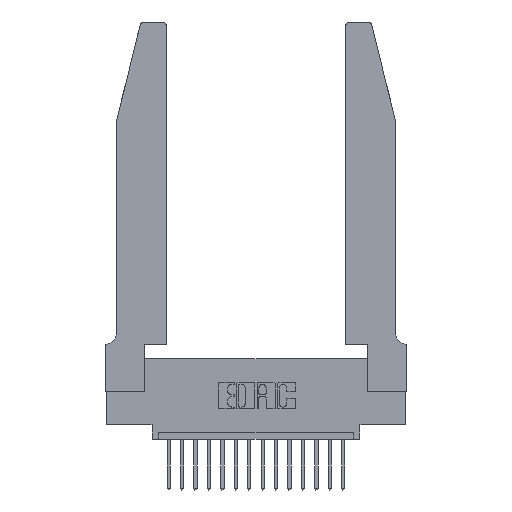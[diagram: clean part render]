
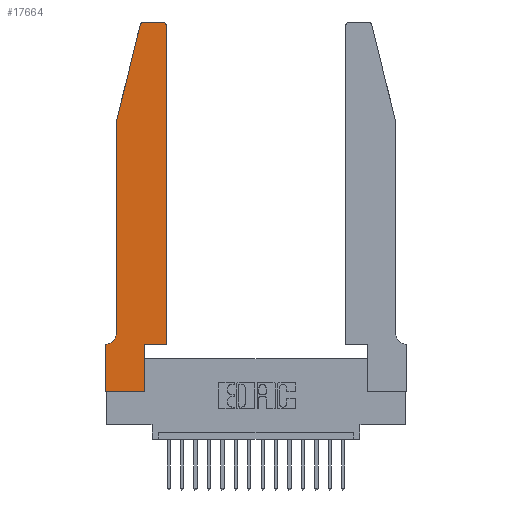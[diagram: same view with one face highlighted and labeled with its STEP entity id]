
A CAD part, top view. The second image highlights one B-rep face of the part: STEP entity #17664.
In plain terms, the highlighted planar face has unit normal (0, 0, 1).
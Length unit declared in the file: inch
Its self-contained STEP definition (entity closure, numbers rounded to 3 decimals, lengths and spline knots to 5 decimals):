
#41 = CARTESIAN_POINT ( 'NONE',  ( 0.0055, 0.35, 0.37 ) ) ;
#336 = DIRECTION ( 'NONE',  ( -1., 0., 0. ) ) ;
#634 = EDGE_CURVE ( 'NONE', #5556, #18562, #10754, .T. ) ;
#783 = EDGE_CURVE ( 'NONE', #3052, #7503, #3589, .T. ) ;
#877 = VECTOR ( 'NONE', #18525, 39.37008 ) ;
#1016 = EDGE_CURVE ( 'NONE', #6034, #7472, #14164, .T. ) ;
#1165 = AXIS2_PLACEMENT_3D ( 'NONE', #6906, #19203, #2947 ) ;
#1180 = VERTEX_POINT ( 'NONE', #10455 ) ;
#1597 = PLANE ( 'NONE',  #2873 ) ;
#2006 = CARTESIAN_POINT ( 'NONE',  ( 0.284, 2.75, 0.37 ) ) ;
#2353 = CARTESIAN_POINT ( 'NONE',  ( 0.0755, 0.35, 0.37 ) ) ;
#2873 = AXIS2_PLACEMENT_3D ( 'NONE', #10588, #7543, #12049 ) ;
#2898 = CARTESIAN_POINT ( 'NONE',  ( 0.2865, 0.35, 0.37 ) ) ;
#2947 = DIRECTION ( 'NONE',  ( -1., 0., 0. ) ) ;
#3052 = VERTEX_POINT ( 'NONE', #2898 ) ;
#3053 = LINE ( 'NONE', #6545, #18101 ) ;
#3283 = ORIENTED_EDGE ( 'NONE', *, *, #8863, .T. ) ;
#3589 = LINE ( 'NONE', #14506, #14929 ) ;
#3853 = VERTEX_POINT ( 'NONE', #41 ) ;
#4022 = CARTESIAN_POINT ( 'NONE',  ( 0.0755, 2., 0.37 ) ) ;
#4273 = CARTESIAN_POINT ( 'NONE',  ( 0.284, 2.72, 0.37 ) ) ;
#4688 = CARTESIAN_POINT ( 'NONE',  ( 0.4205, 2.72, 0.37 ) ) ;
#4776 = VERTEX_POINT ( 'NONE', #8420 ) ;
#4938 = VECTOR ( 'NONE', #336, 39.37008 ) ;
#4961 = ORIENTED_EDGE ( 'NONE', *, *, #18572, .T. ) ;
#5271 = CARTESIAN_POINT ( 'NONE',  ( 0., 0., 0.37 ) ) ;
#5556 = VERTEX_POINT ( 'NONE', #6150 ) ;
#5562 = CARTESIAN_POINT ( 'NONE',  ( 0., 0., 0.37 ) ) ;
#5880 = DIRECTION ( 'NONE',  ( 0., -1., 0. ) ) ;
#5937 = ORIENTED_EDGE ( 'NONE', *, *, #13167, .T. ) ;
#5942 = CARTESIAN_POINT ( 'NONE',  ( 0.0755, 2., 0.37 ) ) ;
#6018 = DIRECTION ( 'NONE',  ( 0., 0., 1. ) ) ;
#6034 = VERTEX_POINT ( 'NONE', #2006 ) ;
#6150 = CARTESIAN_POINT ( 'NONE',  ( 0., 0.35, 0.37 ) ) ;
#6298 = EDGE_CURVE ( 'NONE', #7503, #12622, #3053, .T. ) ;
#6530 = LINE ( 'NONE', #19171, #12340 ) ;
#6545 = CARTESIAN_POINT ( 'NONE',  ( 0.4505, 0.35, 0.37 ) ) ;
#6712 = DIRECTION ( 'NONE',  ( -0.239, -0.971, 0. ) ) ;
#6735 = EDGE_CURVE ( 'NONE', #3853, #5556, #12672, .T. ) ;
#6906 = CARTESIAN_POINT ( 'NONE',  ( 0.0055, 0.42, 0.37 ) ) ;
#6975 = DIRECTION ( 'NONE',  ( 0., -1., 0. ) ) ;
#7262 = VERTEX_POINT ( 'NONE', #4022 ) ;
#7472 = VERTEX_POINT ( 'NONE', #16097 ) ;
#7503 = VERTEX_POINT ( 'NONE', #11433 ) ;
#7543 = DIRECTION ( 'NONE',  ( 0., 0., 1. ) ) ;
#8420 = CARTESIAN_POINT ( 'NONE',  ( 0.2865, 0., 0.37 ) ) ;
#8599 = VERTEX_POINT ( 'NONE', #8925 ) ;
#8727 = DIRECTION ( 'NONE',  ( 1., 0., 0. ) ) ;
#8863 = EDGE_CURVE ( 'NONE', #12622, #1180, #12845, .T. ) ;
#8875 = LINE ( 'NONE', #13602, #4938 ) ;
#8925 = CARTESIAN_POINT ( 'NONE',  ( 0.0755, 0.42, 0.37 ) ) ;
#9743 = DIRECTION ( 'NONE',  ( 1., 0., 0. ) ) ;
#10354 = EDGE_CURVE ( 'NONE', #4776, #3052, #6530, .T. ) ;
#10398 = LINE ( 'NONE', #5271, #12910 ) ;
#10455 = CARTESIAN_POINT ( 'NONE',  ( 0.4205, 2.75, 0.37 ) ) ;
#10588 = CARTESIAN_POINT ( 'NONE',  ( 0., 0.35, 0.37 ) ) ;
#10690 = ORIENTED_EDGE ( 'NONE', *, *, #634, .T. ) ;
#10738 = CARTESIAN_POINT ( 'NONE',  ( 0., 0., 0.37 ) ) ;
#10754 = LINE ( 'NONE', #5562, #17048 ) ;
#11433 = CARTESIAN_POINT ( 'NONE',  ( 0.4505, 0.35, 0.37 ) ) ;
#11901 = DIRECTION ( 'NONE',  ( 1., 0., 0. ) ) ;
#12049 = DIRECTION ( 'NONE',  ( 1., 0., 0. ) ) ;
#12340 = VECTOR ( 'NONE', #14731, 39.37008 ) ;
#12451 = CIRCLE ( 'NONE', #1165, 0.07 ) ;
#12622 = VERTEX_POINT ( 'NONE', #17274 ) ;
#12647 = LINE ( 'NONE', #5942, #15228 ) ;
#12672 = LINE ( 'NONE', #2353, #877 ) ;
#12845 = CIRCLE ( 'NONE', #16046, 0.03 ) ;
#12910 = VECTOR ( 'NONE', #9743, 39.37008 ) ;
#12934 = EDGE_CURVE ( 'NONE', #7472, #7262, #13156, .T. ) ;
#13156 = LINE ( 'NONE', #14064, #18993 ) ;
#13167 = EDGE_CURVE ( 'NONE', #8599, #3853, #12451, .T. ) ;
#13602 = CARTESIAN_POINT ( 'NONE',  ( 0.2605, 2.75, 0.37 ) ) ;
#14064 = CARTESIAN_POINT ( 'NONE',  ( 0.0755, 2., 0.37 ) ) ;
#14164 = CIRCLE ( 'NONE', #15677, 0.03 ) ;
#14249 = EDGE_CURVE ( 'NONE', #18562, #4776, #10398, .T. ) ;
#14506 = CARTESIAN_POINT ( 'NONE',  ( 0.4505, 0.35, 0.37 ) ) ;
#14731 = DIRECTION ( 'NONE',  ( 0., 1., 0. ) ) ;
#14807 = ORIENTED_EDGE ( 'NONE', *, *, #14249, .T. ) ;
#14929 = VECTOR ( 'NONE', #16043, 39.37008 ) ;
#14943 = ORIENTED_EDGE ( 'NONE', *, *, #12934, .T. ) ;
#15165 = EDGE_CURVE ( 'NONE', #7262, #8599, #12647, .T. ) ;
#15228 = VECTOR ( 'NONE', #5880, 39.37008 ) ;
#15275 = ORIENTED_EDGE ( 'NONE', *, *, #6735, .T. ) ;
#15677 = AXIS2_PLACEMENT_3D ( 'NONE', #4273, #16148, #8727 ) ;
#15789 = ORIENTED_EDGE ( 'NONE', *, *, #783, .T. ) ;
#15875 = ORIENTED_EDGE ( 'NONE', *, *, #6298, .T. ) ;
#16043 = DIRECTION ( 'NONE',  ( 1., 0., 0. ) ) ;
#16046 = AXIS2_PLACEMENT_3D ( 'NONE', #4688, #6018, #11901 ) ;
#16097 = CARTESIAN_POINT ( 'NONE',  ( 0.25487, 2.72718, 0.37 ) ) ;
#16148 = DIRECTION ( 'NONE',  ( 0., 0., 1. ) ) ;
#16701 = ORIENTED_EDGE ( 'NONE', *, *, #10354, .T. ) ;
#16963 = DIRECTION ( 'NONE',  ( 0., 1., 0. ) ) ;
#17048 = VECTOR ( 'NONE', #6975, 39.37008 ) ;
#17274 = CARTESIAN_POINT ( 'NONE',  ( 0.4505, 2.72, 0.37 ) ) ;
#17664 = ADVANCED_FACE ( 'NONE', ( #18397 ), #1597, .T. ) ;
#18101 = VECTOR ( 'NONE', #16963, 39.37008 ) ;
#18397 = FACE_OUTER_BOUND ( 'NONE', #18878, .T. ) ;
#18525 = DIRECTION ( 'NONE',  ( -1., 0., 0. ) ) ;
#18562 = VERTEX_POINT ( 'NONE', #10738 ) ;
#18572 = EDGE_CURVE ( 'NONE', #1180, #6034, #8875, .T. ) ;
#18693 = ORIENTED_EDGE ( 'NONE', *, *, #1016, .T. ) ;
#18878 = EDGE_LOOP ( 'NONE', ( #4961, #18693, #14943, #18946, #5937, #15275, #10690, #14807, #16701, #15789, #15875, #3283 ) ) ;
#18946 = ORIENTED_EDGE ( 'NONE', *, *, #15165, .T. ) ;
#18993 = VECTOR ( 'NONE', #6712, 39.37008 ) ;
#19171 = CARTESIAN_POINT ( 'NONE',  ( 0.2865, 0.35, 0.37 ) ) ;
#19203 = DIRECTION ( 'NONE',  ( 0., 0., -1. ) ) ;
